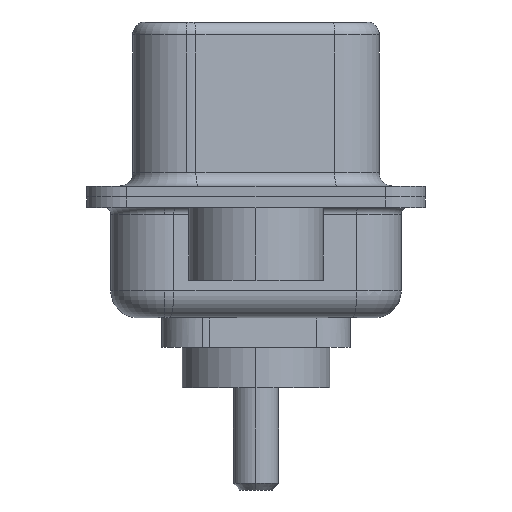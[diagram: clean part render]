
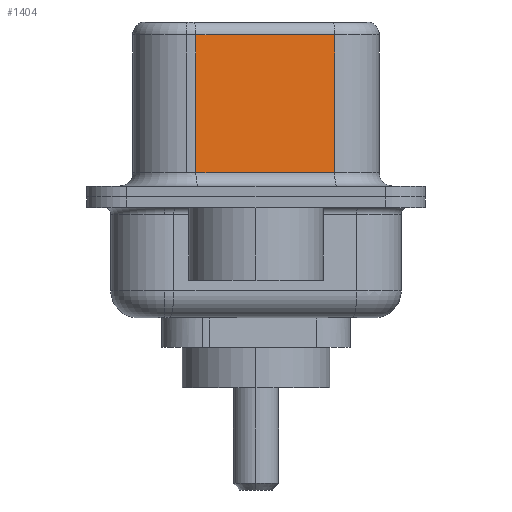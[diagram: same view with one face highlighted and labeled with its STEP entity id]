
A CAD part, left-side view. The second image highlights one B-rep face of the part: STEP entity #1404.
In plain terms, the highlighted planar face has unit normal (-0.985, -0.174, 0).
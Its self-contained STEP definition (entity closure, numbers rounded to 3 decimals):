
#311 = LINE ( 'NONE', #2716, #11120 ) ;
#965 = EDGE_CURVE ( 'NONE', #11096, #9778, #311, .T. ) ;
#1155 = LINE ( 'NONE', #2677, #15284 ) ;
#1404 = ADVANCED_FACE ( 'NONE', ( #9535 ), #1729, .F. ) ;
#1729 = PLANE ( 'NONE',  #4627 ) ;
#1984 = DIRECTION ( 'NONE',  ( 0.174, -0.985, 0. ) ) ;
#2677 = CARTESIAN_POINT ( 'NONE',  ( 3.655, 2.233, 6.52 ) ) ;
#2716 = CARTESIAN_POINT ( 'NONE',  ( 4.565, -2.927, 6.52 ) ) ;
#2934 = VECTOR ( 'NONE', #12790, 1000. ) ;
#4380 = CARTESIAN_POINT ( 'NONE',  ( 4.565, -2.927, 6.02 ) ) ;
#4627 = AXIS2_PLACEMENT_3D ( 'NONE', #11922, #11480, #8474 ) ;
#5665 = CARTESIAN_POINT ( 'NONE',  ( 4.565, -2.927, 6.02 ) ) ;
#6180 = LINE ( 'NONE', #4380, #2934 ) ;
#6729 = VERTEX_POINT ( 'NONE', #16366 ) ;
#8474 = DIRECTION ( 'NONE',  ( -0.174, 0.985, 0. ) ) ;
#8933 = EDGE_CURVE ( 'NONE', #11096, #6729, #6180, .T. ) ;
#9072 = CARTESIAN_POINT ( 'NONE',  ( 3.655, 2.233, 0.9 ) ) ;
#9180 = EDGE_CURVE ( 'NONE', #15372, #9778, #10183, .T. ) ;
#9535 = FACE_OUTER_BOUND ( 'NONE', #16467, .T. ) ;
#9778 = VERTEX_POINT ( 'NONE', #11574 ) ;
#10183 = LINE ( 'NONE', #13221, #13910 ) ;
#10190 = ORIENTED_EDGE ( 'NONE', *, *, #18308, .T. ) ;
#11096 = VERTEX_POINT ( 'NONE', #5665 ) ;
#11120 = VECTOR ( 'NONE', #15389, 1000. ) ;
#11480 = DIRECTION ( 'NONE',  ( 0.985, 0.174, 0. ) ) ;
#11574 = CARTESIAN_POINT ( 'NONE',  ( 4.565, -2.927, 0.9 ) ) ;
#11922 = CARTESIAN_POINT ( 'NONE',  ( 4.565, -2.927, 6.52 ) ) ;
#12036 = ORIENTED_EDGE ( 'NONE', *, *, #965, .F. ) ;
#12501 = DIRECTION ( 'NONE',  ( 0., 0., -1. ) ) ;
#12790 = DIRECTION ( 'NONE',  ( -0.174, 0.985, 0. ) ) ;
#13197 = ORIENTED_EDGE ( 'NONE', *, *, #8933, .T. ) ;
#13221 = CARTESIAN_POINT ( 'NONE',  ( 4.565, -2.927, 0.9 ) ) ;
#13910 = VECTOR ( 'NONE', #1984, 1000. ) ;
#13940 = ORIENTED_EDGE ( 'NONE', *, *, #9180, .T. ) ;
#15284 = VECTOR ( 'NONE', #12501, 1000. ) ;
#15372 = VERTEX_POINT ( 'NONE', #9072 ) ;
#15389 = DIRECTION ( 'NONE',  ( 0., 0., -1. ) ) ;
#16366 = CARTESIAN_POINT ( 'NONE',  ( 3.655, 2.233, 6.02 ) ) ;
#16467 = EDGE_LOOP ( 'NONE', ( #12036, #13197, #10190, #13940 ) ) ;
#18308 = EDGE_CURVE ( 'NONE', #6729, #15372, #1155, .T. ) ;
